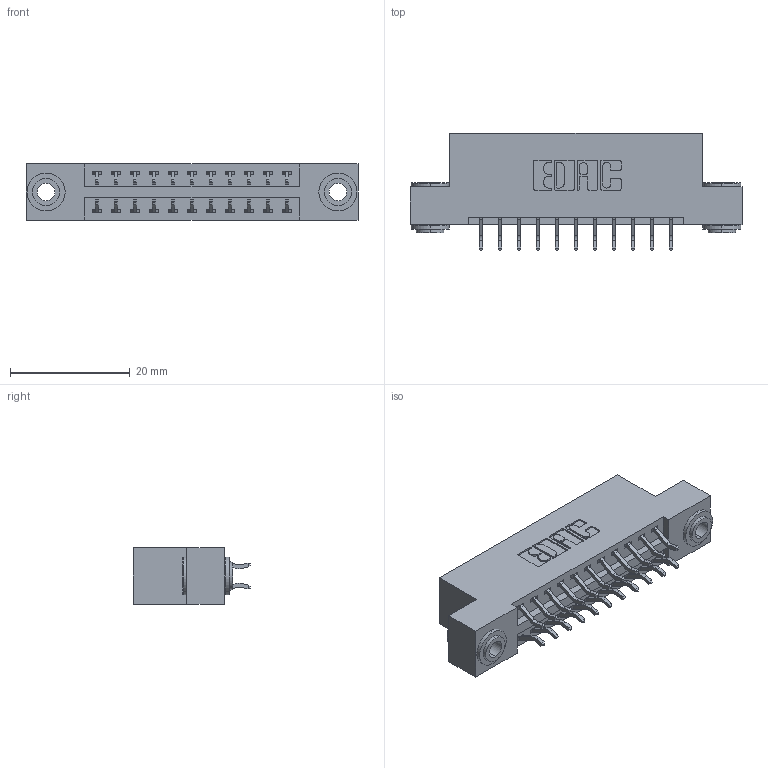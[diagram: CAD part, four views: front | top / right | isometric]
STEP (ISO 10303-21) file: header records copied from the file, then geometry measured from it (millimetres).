
FILE_DESCRIPTION (( 'STEP AP203' ), '1' );
FILE_NAME ('396-022-556-203.STEP', '2019-10-30T03:57:01', ( '' ), ( '' ), 'SwSTEP 2.0', 'SolidWorks 2016', '' );
FILE_SCHEMA (( 'CONFIG_CONTROL_DESIGN' ));
Length unit declared in the file: inch
Products named in the file (4): 345-250-002_345-250-002-102; 345-292-001_556 Tail; 346 Part_Flush Mounting Lugs - 0.156 Dia-TH; 396-022-556-203
Assembly tree (25 placements, depth 2):
  396-022-556-203
    346 Part_Flush Mounting Lugs - 0.156 Dia-TH
    345-292-001_556 Tail  x22
    345-250-002_345-250-002-102  x2
Bounding box: 55.5 x 19.57 x 9.4 mm (x, y, z)
Volume: 5189.6 mm3; surface area: 6839.9 mm2
Topology: 25 solids, 25 shells, 1436 faces, 4211 edges, 2774 vertices
Faces by surface type: plane 944, cylinder 484, cone 8
Entity records: 12222 total; most frequent: CARTESIAN_POINT 2047, ORIENTED_EDGE 1962, DIRECTION 1875, EDGE_CURVE 981, LINE 773, VECTOR 773, VERTEX_POINT 650, AXIS2_PLACEMENT_3D 551
